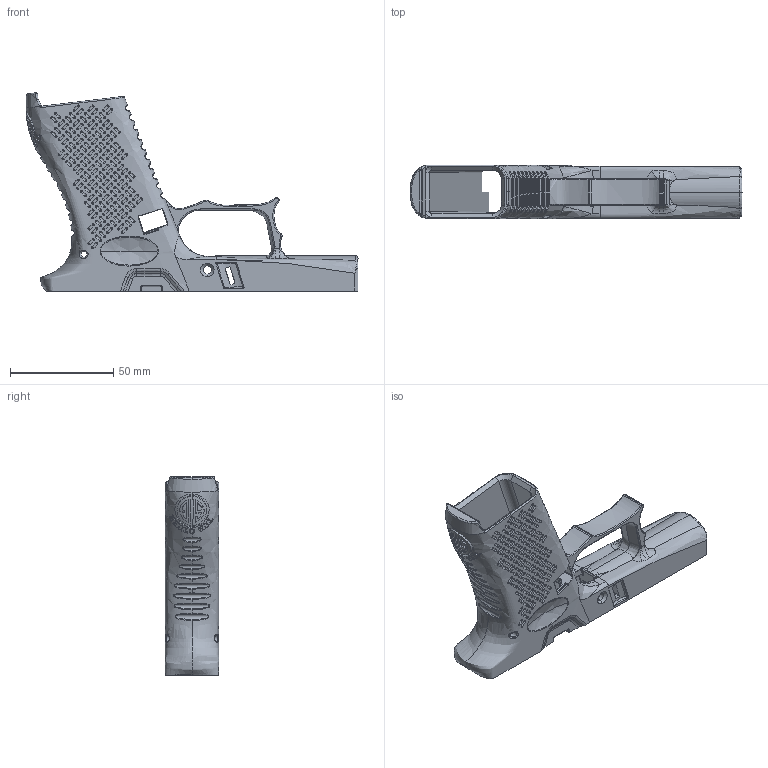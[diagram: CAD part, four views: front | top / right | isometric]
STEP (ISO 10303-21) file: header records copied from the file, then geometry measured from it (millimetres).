
FILE_DESCRIPTION (( 'STEP AP203' ), '1' );
FILE_NAME ('43X BasketWeave FDM.STEP', '2020-12-17T01:35:42', ( '' ), ( '' ), 'SwSTEP 2.0', 'SolidWorks 2016', '' );
FILE_SCHEMA (( 'CONFIG_CONTROL_DESIGN' ));
Products named in the file (1): 43X BasketWeave FDM
Bounding box: 160.56 x 25.9 x 95.92 mm (x, y, z)
Volume: 63009 mm3; surface area: 39039.9 mm2
Topology: 1 solids, 1 shells, 2400 faces, 6027 edges, 3872 vertices
Faces by surface type: sphere 821, cylinder 631, bspline 464, plane 446, torus 26, cone 12
Entity records: 122787 total; most frequent: CARTESIAN_POINT 72518, ORIENTED_EDGE 11982, DIRECTION 8048, EDGE_CURVE 5991, VERTEX_POINT 3872, AXIS2_PLACEMENT_3D 3528, B_SPLINE_CURVE_WITH_KNOTS 3302, EDGE_LOOP 2701
